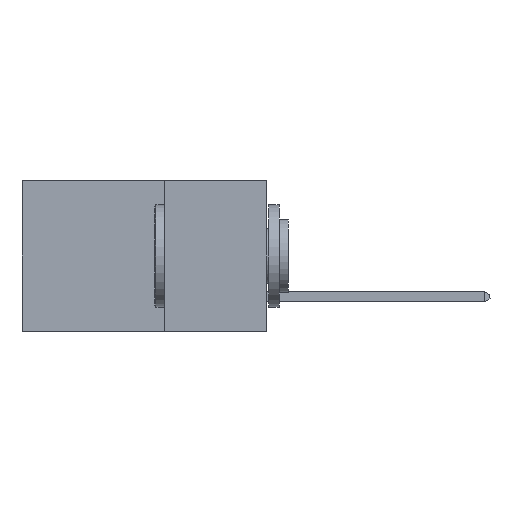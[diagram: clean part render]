
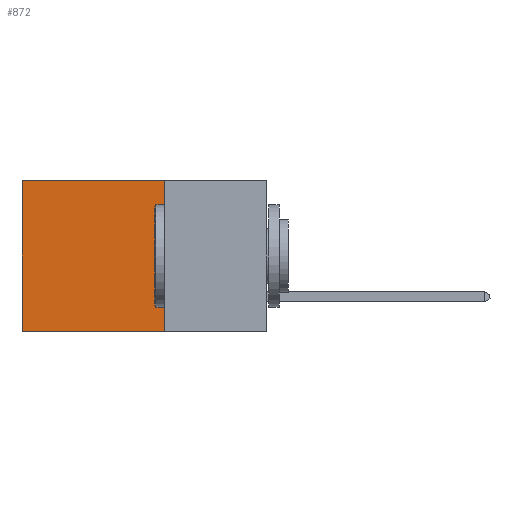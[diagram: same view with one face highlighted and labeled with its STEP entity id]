
A CAD part, left-side view. The second image highlights one B-rep face of the part: STEP entity #872.
In plain terms, the highlighted planar face has unit normal (-1, 0, 0).
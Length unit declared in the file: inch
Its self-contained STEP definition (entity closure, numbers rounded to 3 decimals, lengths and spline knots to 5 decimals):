
#467 = VERTEX_POINT ( 'NONE', #9021 ) ;
#744 = DIRECTION ( 'NONE',  ( 0., 1., 0. ) ) ;
#804 = EDGE_LOOP ( 'NONE', ( #12012, #10292, #4480, #5557 ) ) ;
#872 = ADVANCED_FACE ( 'NONE', ( #4581 ), #10724, .F. ) ;
#1226 = DIRECTION ( 'NONE',  ( 0., 0., -1. ) ) ;
#1588 = LINE ( 'NONE', #10322, #3738 ) ;
#1590 = CARTESIAN_POINT ( 'NONE',  ( 0.2875, 0.6, -0.37 ) ) ;
#2321 = VECTOR ( 'NONE', #744, 39.37008 ) ;
#2763 = DIRECTION ( 'NONE',  ( 0., 1., 0. ) ) ;
#3715 = AXIS2_PLACEMENT_3D ( 'NONE', #4392, #5451, #1226 ) ;
#3738 = VECTOR ( 'NONE', #2763, 39.37008 ) ;
#3999 = EDGE_CURVE ( 'NONE', #11881, #467, #1588, .T. ) ;
#4341 = CARTESIAN_POINT ( 'NONE',  ( 0.2875, 0.25, -0.37 ) ) ;
#4372 = CARTESIAN_POINT ( 'NONE',  ( 0.2875, 0.25, 0. ) ) ;
#4392 = CARTESIAN_POINT ( 'NONE',  ( 0.2875, 0.25, 0. ) ) ;
#4480 = ORIENTED_EDGE ( 'NONE', *, *, #8541, .F. ) ;
#4581 = FACE_OUTER_BOUND ( 'NONE', #804, .T. ) ;
#4856 = DIRECTION ( 'NONE',  ( 0., 0., -1. ) ) ;
#5451 = DIRECTION ( 'NONE',  ( 1., 0., 0. ) ) ;
#5557 = ORIENTED_EDGE ( 'NONE', *, *, #3999, .T. ) ;
#5755 = LINE ( 'NONE', #4372, #8748 ) ;
#7225 = CARTESIAN_POINT ( 'NONE',  ( 0.2875, 0.25, -0.37 ) ) ;
#8065 = CARTESIAN_POINT ( 'NONE',  ( 0.2875, 0.6, 0. ) ) ;
#8335 = VERTEX_POINT ( 'NONE', #4341 ) ;
#8487 = VECTOR ( 'NONE', #4856, 39.37008 ) ;
#8541 = EDGE_CURVE ( 'NONE', #11881, #8335, #5755, .T. ) ;
#8748 = VECTOR ( 'NONE', #11776, 39.37008 ) ;
#9021 = CARTESIAN_POINT ( 'NONE',  ( 0.2875, 0.6, 0. ) ) ;
#10292 = ORIENTED_EDGE ( 'NONE', *, *, #12000, .F. ) ;
#10322 = CARTESIAN_POINT ( 'NONE',  ( 0.2875, 0.25, 0. ) ) ;
#10530 = CARTESIAN_POINT ( 'NONE',  ( 0.2875, 0.25, 0. ) ) ;
#10724 = PLANE ( 'NONE',  #3715 ) ;
#11086 = LINE ( 'NONE', #8065, #8487 ) ;
#11776 = DIRECTION ( 'NONE',  ( 0., 0., -1. ) ) ;
#11881 = VERTEX_POINT ( 'NONE', #10530 ) ;
#12000 = EDGE_CURVE ( 'NONE', #8335, #12910, #12600, .T. ) ;
#12012 = ORIENTED_EDGE ( 'NONE', *, *, #12306, .T. ) ;
#12306 = EDGE_CURVE ( 'NONE', #467, #12910, #11086, .T. ) ;
#12600 = LINE ( 'NONE', #7225, #2321 ) ;
#12910 = VERTEX_POINT ( 'NONE', #1590 ) ;
